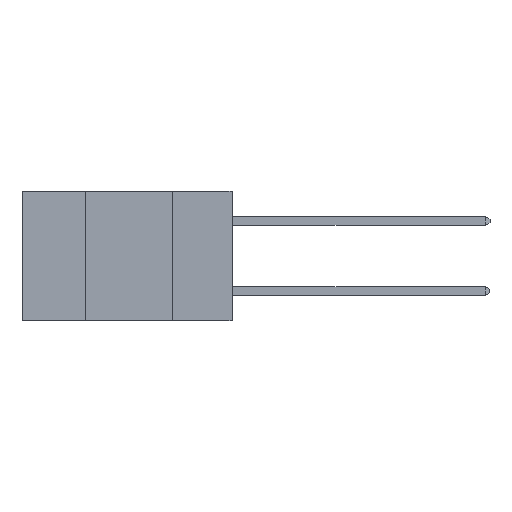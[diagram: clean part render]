
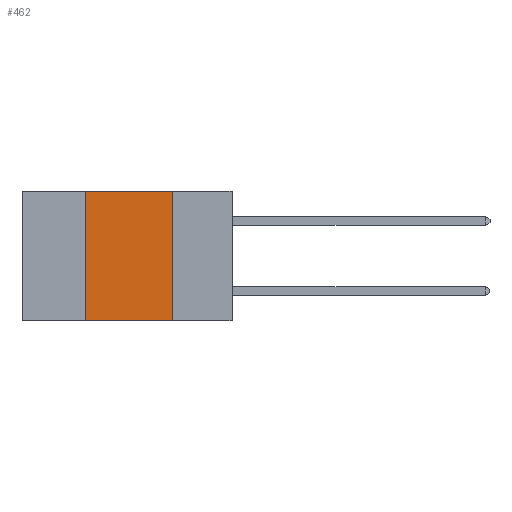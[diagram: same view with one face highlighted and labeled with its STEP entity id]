
A CAD part, left-side view. The second image highlights one B-rep face of the part: STEP entity #462.
In plain terms, the highlighted planar face has unit normal (-1, 0, 0).
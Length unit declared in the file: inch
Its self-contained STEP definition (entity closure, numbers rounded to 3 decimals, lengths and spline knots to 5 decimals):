
#6 = EDGE_CURVE ( 'NONE', #380, #15290, #7174, .T. ) ;
#380 = VERTEX_POINT ( 'NONE', #2817 ) ;
#447 = VECTOR ( 'NONE', #2929, 39.37008 ) ;
#462 = ADVANCED_FACE ( 'NONE', ( #12162 ), #1299, .F. ) ;
#543 = DIRECTION ( 'NONE',  ( 1., 0., 0. ) ) ;
#657 = AXIS2_PLACEMENT_3D ( 'NONE', #4185, #543, #11165 ) ;
#1012 = VECTOR ( 'NONE', #14506, 39.37008 ) ;
#1299 = PLANE ( 'NONE',  #657 ) ;
#1428 = LINE ( 'NONE', #13344, #1012 ) ;
#1995 = CARTESIAN_POINT ( 'NONE',  ( 0., 0.42, -0.37 ) ) ;
#2408 = LINE ( 'NONE', #10675, #8564 ) ;
#2789 = EDGE_CURVE ( 'NONE', #9276, #12197, #2408, .T. ) ;
#2817 = CARTESIAN_POINT ( 'NONE',  ( 0., 0.42, 0. ) ) ;
#2883 = EDGE_CURVE ( 'NONE', #15290, #12197, #3839, .T. ) ;
#2929 = DIRECTION ( 'NONE',  ( 0., 0., -1. ) ) ;
#3839 = LINE ( 'NONE', #9745, #447 ) ;
#3980 = VECTOR ( 'NONE', #9947, 39.37008 ) ;
#4185 = CARTESIAN_POINT ( 'NONE',  ( 0., 0.6, 0. ) ) ;
#5557 = ORIENTED_EDGE ( 'NONE', *, *, #6, .F. ) ;
#5946 = CARTESIAN_POINT ( 'NONE',  ( 0., 0.17, 0. ) ) ;
#6612 = EDGE_CURVE ( 'NONE', #9276, #380, #1428, .T. ) ;
#7174 = LINE ( 'NONE', #14794, #3980 ) ;
#7561 = EDGE_LOOP ( 'NONE', ( #9518, #5557, #7857, #14761 ) ) ;
#7857 = ORIENTED_EDGE ( 'NONE', *, *, #6612, .F. ) ;
#8564 = VECTOR ( 'NONE', #9941, 39.37008 ) ;
#9276 = VERTEX_POINT ( 'NONE', #1995 ) ;
#9518 = ORIENTED_EDGE ( 'NONE', *, *, #2883, .F. ) ;
#9745 = CARTESIAN_POINT ( 'NONE',  ( 0., 0.17, 0. ) ) ;
#9941 = DIRECTION ( 'NONE',  ( 0., -1., 0. ) ) ;
#9947 = DIRECTION ( 'NONE',  ( 0., -1., 0. ) ) ;
#10675 = CARTESIAN_POINT ( 'NONE',  ( 0., 0.6, -0.37 ) ) ;
#11110 = CARTESIAN_POINT ( 'NONE',  ( 0., 0.17, -0.37 ) ) ;
#11165 = DIRECTION ( 'NONE',  ( 0., 0., -1. ) ) ;
#12162 = FACE_OUTER_BOUND ( 'NONE', #7561, .T. ) ;
#12197 = VERTEX_POINT ( 'NONE', #11110 ) ;
#13344 = CARTESIAN_POINT ( 'NONE',  ( 0., 0.42, 0. ) ) ;
#14506 = DIRECTION ( 'NONE',  ( 0., 0., 1. ) ) ;
#14761 = ORIENTED_EDGE ( 'NONE', *, *, #2789, .T. ) ;
#14794 = CARTESIAN_POINT ( 'NONE',  ( 0., 0.6, 0. ) ) ;
#15290 = VERTEX_POINT ( 'NONE', #5946 ) ;
